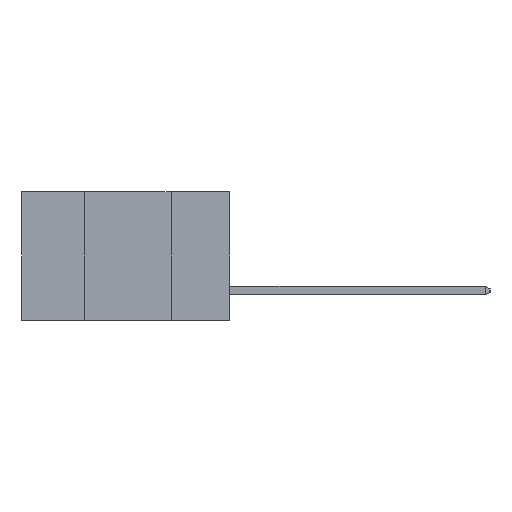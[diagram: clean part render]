
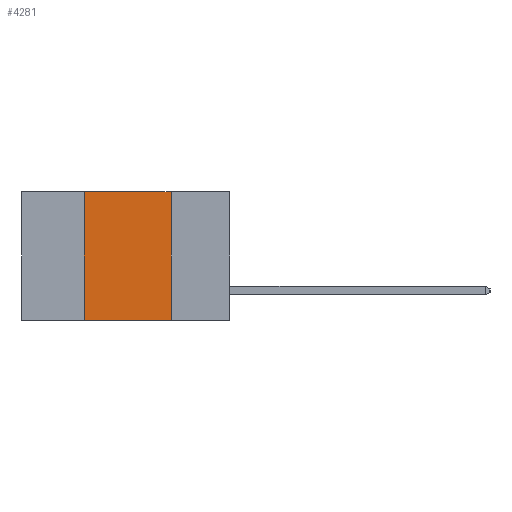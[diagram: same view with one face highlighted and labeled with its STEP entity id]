
A CAD part, left-side view. The second image highlights one B-rep face of the part: STEP entity #4281.
In plain terms, the highlighted planar face has unit normal (-1, 0, 0).
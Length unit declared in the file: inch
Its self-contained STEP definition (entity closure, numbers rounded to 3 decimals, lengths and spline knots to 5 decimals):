
#1795 = CARTESIAN_POINT ( 'NONE',  ( 0., 0.17, 0. ) ) ;
#2098 = CARTESIAN_POINT ( 'NONE',  ( 0., 0.42, 0. ) ) ;
#2302 = VERTEX_POINT ( 'NONE', #16540 ) ;
#2338 = VERTEX_POINT ( 'NONE', #16646 ) ;
#3918 = ORIENTED_EDGE ( 'NONE', *, *, #12990, .T. ) ;
#4281 = ADVANCED_FACE ( 'NONE', ( #19875 ), #5035, .F. ) ;
#4532 = LINE ( 'NONE', #24229, #23014 ) ;
#4970 = DIRECTION ( 'NONE',  ( 0., 0., 1. ) ) ;
#5035 = PLANE ( 'NONE',  #11937 ) ;
#5055 = VECTOR ( 'NONE', #10924, 39.37008 ) ;
#7476 = DIRECTION ( 'NONE',  ( 0., 0., -1. ) ) ;
#8563 = CARTESIAN_POINT ( 'NONE',  ( 0., 0.6, -0.37 ) ) ;
#10924 = DIRECTION ( 'NONE',  ( 0., -1., 0. ) ) ;
#11094 = VERTEX_POINT ( 'NONE', #1795 ) ;
#11183 = VERTEX_POINT ( 'NONE', #2098 ) ;
#11689 = VECTOR ( 'NONE', #14551, 39.37008 ) ;
#11937 = AXIS2_PLACEMENT_3D ( 'NONE', #17055, #21863, #7476 ) ;
#12382 = LINE ( 'NONE', #14391, #30722 ) ;
#12990 = EDGE_CURVE ( 'NONE', #2302, #2338, #24254, .T. ) ;
#14391 = CARTESIAN_POINT ( 'NONE',  ( 0., 0.6, 0. ) ) ;
#14551 = DIRECTION ( 'NONE',  ( 0., 0., -1. ) ) ;
#15696 = ORIENTED_EDGE ( 'NONE', *, *, #29603, .F. ) ;
#16540 = CARTESIAN_POINT ( 'NONE',  ( 0., 0.42, -0.37 ) ) ;
#16646 = CARTESIAN_POINT ( 'NONE',  ( 0., 0.17, -0.37 ) ) ;
#17055 = CARTESIAN_POINT ( 'NONE',  ( 0., 0.6, 0. ) ) ;
#19329 = CARTESIAN_POINT ( 'NONE',  ( 0., 0.17, 0. ) ) ;
#19875 = FACE_OUTER_BOUND ( 'NONE', #23052, .T. ) ;
#21574 = EDGE_CURVE ( 'NONE', #11094, #2338, #25175, .T. ) ;
#21863 = DIRECTION ( 'NONE',  ( 1., 0., 0. ) ) ;
#23014 = VECTOR ( 'NONE', #4970, 39.37008 ) ;
#23052 = EDGE_LOOP ( 'NONE', ( #23334, #24271, #15696, #3918 ) ) ;
#23064 = EDGE_CURVE ( 'NONE', #11183, #11094, #12382, .T. ) ;
#23334 = ORIENTED_EDGE ( 'NONE', *, *, #21574, .F. ) ;
#24229 = CARTESIAN_POINT ( 'NONE',  ( 0., 0.42, 0. ) ) ;
#24254 = LINE ( 'NONE', #8563, #5055 ) ;
#24271 = ORIENTED_EDGE ( 'NONE', *, *, #23064, .F. ) ;
#25175 = LINE ( 'NONE', #19329, #11689 ) ;
#26339 = DIRECTION ( 'NONE',  ( 0., -1., 0. ) ) ;
#29603 = EDGE_CURVE ( 'NONE', #2302, #11183, #4532, .T. ) ;
#30722 = VECTOR ( 'NONE', #26339, 39.37008 ) ;
